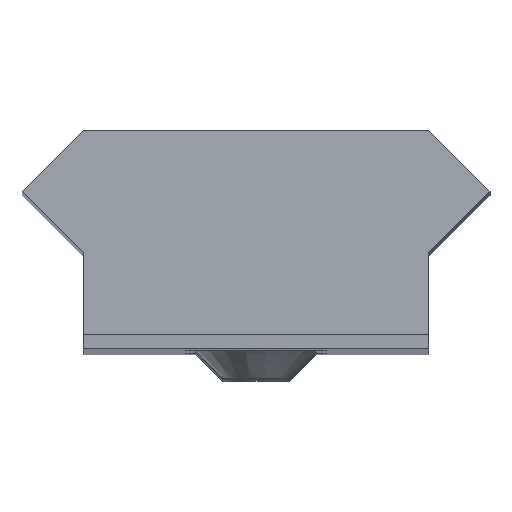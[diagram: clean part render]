
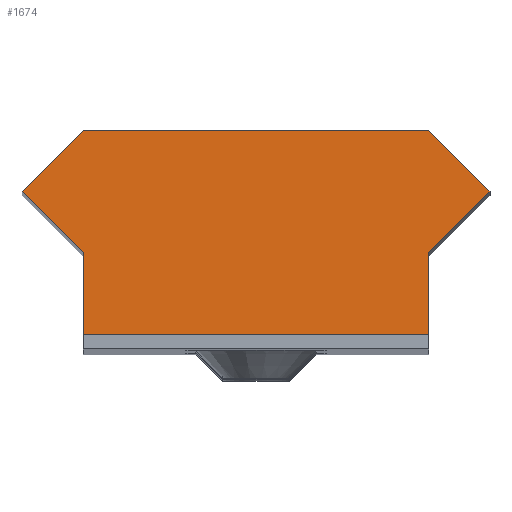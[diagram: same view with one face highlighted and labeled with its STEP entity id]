
A CAD part, top view. The second image highlights one B-rep face of the part: STEP entity #1674.
In plain terms, the highlighted planar face has unit normal (0, 0.939, 0.344).
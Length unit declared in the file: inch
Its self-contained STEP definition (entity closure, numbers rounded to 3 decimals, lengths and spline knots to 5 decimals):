
#103=PLANE('',#1829);
#196=FACE_OUTER_BOUND('',#298,.T.);
#298=EDGE_LOOP('',(#1529,#1530,#1531,#1532,#1533,#1534,#1535,#1536));
#310=LINE('',#2329,#502);
#336=LINE('',#2458,#528);
#474=LINE('',#2732,#666);
#477=LINE('',#2737,#669);
#478=LINE('',#2740,#670);
#481=LINE('',#2745,#673);
#488=LINE('',#2759,#680);
#489=LINE('',#2760,#681);
#502=VECTOR('',#1865,0.3937);
#528=VECTOR('',#1991,0.3937);
#666=VECTOR('',#2257,0.3937);
#669=VECTOR('',#2262,0.3937);
#670=VECTOR('',#2265,0.3937);
#673=VECTOR('',#2270,0.3937);
#680=VECTOR('',#2283,0.3937);
#681=VECTOR('',#2284,0.3937);
#739=VERTEX_POINT('',#2327);
#740=VERTEX_POINT('',#2328);
#792=VERTEX_POINT('',#2455);
#793=VERTEX_POINT('',#2457);
#865=VERTEX_POINT('',#2731);
#866=VERTEX_POINT('',#2735);
#867=VERTEX_POINT('',#2739);
#872=VERTEX_POINT('',#2758);
#888=EDGE_CURVE('',#739,#740,#310,.T.);
#950=EDGE_CURVE('',#792,#793,#336,.T.);
#1088=EDGE_CURVE('',#793,#865,#474,.T.);
#1091=EDGE_CURVE('',#866,#792,#477,.T.);
#1092=EDGE_CURVE('',#740,#867,#478,.T.);
#1095=EDGE_CURVE('',#867,#866,#481,.T.);
#1102=EDGE_CURVE('',#872,#739,#488,.T.);
#1103=EDGE_CURVE('',#865,#872,#489,.T.);
#1529=ORIENTED_EDGE('',*,*,#1102,.F.);
#1530=ORIENTED_EDGE('',*,*,#1103,.F.);
#1531=ORIENTED_EDGE('',*,*,#1088,.F.);
#1532=ORIENTED_EDGE('',*,*,#950,.F.);
#1533=ORIENTED_EDGE('',*,*,#1091,.F.);
#1534=ORIENTED_EDGE('',*,*,#1095,.F.);
#1535=ORIENTED_EDGE('',*,*,#1092,.F.);
#1536=ORIENTED_EDGE('',*,*,#888,.F.);
#1674=ADVANCED_FACE('',(#196),#103,.T.);
#1829=AXIS2_PLACEMENT_3D('',#2757,#2281,#2282);
#1865=DIRECTION('',(-1.,0.,0.));
#1991=DIRECTION('',(1.,0.,0.));
#2257=DIRECTION('',(0.325,-0.325,0.888));
#2262=DIRECTION('',(0.325,0.325,-0.888));
#2265=DIRECTION('',(0.,0.344,-0.939));
#2270=DIRECTION('',(-0.325,0.325,-0.888));
#2281=DIRECTION('center_axis',(0.,0.939,0.344));
#2282=DIRECTION('ref_axis',(0.,-0.344,0.939));
#2283=DIRECTION('',(0.,-0.344,0.939));
#2284=DIRECTION('',(-0.325,-0.325,0.888));
#2327=CARTESIAN_POINT('',(0.30846,-0.25728,5.8));
#2328=CARTESIAN_POINT('',(-0.30846,-0.25728,5.8));
#2329=CARTESIAN_POINT('',(0.,-0.25728,5.8));
#2455=CARTESIAN_POINT('',(-0.30846,0.10886,4.8));
#2457=CARTESIAN_POINT('',(0.30846,0.10886,4.8));
#2458=CARTESIAN_POINT('',(0.15423,0.10886,4.8));
#2731=CARTESIAN_POINT('',(0.41732,0.,5.09731));
#2732=CARTESIAN_POINT('',(-0.38928,0.8066,2.89433));
#2735=CARTESIAN_POINT('',(-0.41732,0.,5.09731));
#2737=CARTESIAN_POINT('',(0.38928,0.8066,2.89433));
#2739=CARTESIAN_POINT('',(-0.30846,-0.10886,5.39462));
#2740=CARTESIAN_POINT('',(-0.30846,0.86208,2.74282));
#2745=CARTESIAN_POINT('',(-1.1683,0.75098,3.04626));
#2757=CARTESIAN_POINT('Origin',(0.,0.10886,4.8));
#2758=CARTESIAN_POINT('',(0.30846,-0.10886,5.39462));
#2759=CARTESIAN_POINT('',(0.30846,0.86208,2.74282));
#2760=CARTESIAN_POINT('',(1.1683,0.75098,3.04626));
